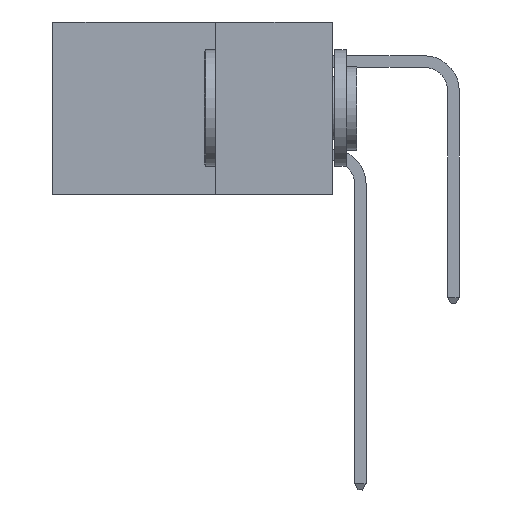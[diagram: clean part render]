
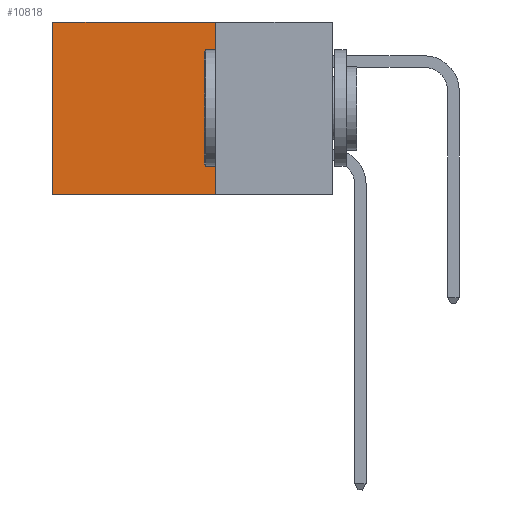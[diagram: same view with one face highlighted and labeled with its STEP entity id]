
A CAD part, left-side view. The second image highlights one B-rep face of the part: STEP entity #10818.
In plain terms, the highlighted planar face has unit normal (-1, 0, 0).
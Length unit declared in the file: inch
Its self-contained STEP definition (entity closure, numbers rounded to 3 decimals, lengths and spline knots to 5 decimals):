
#80 = VERTEX_POINT ( 'NONE', #12510 ) ;
#536 = FACE_OUTER_BOUND ( 'NONE', #19114, .T. ) ;
#728 = ORIENTED_EDGE ( 'NONE', *, *, #16095, .F. ) ;
#775 = VERTEX_POINT ( 'NONE', #17365 ) ;
#1237 = DIRECTION ( 'NONE',  ( 0., 0., -1. ) ) ;
#1368 = VECTOR ( 'NONE', #24370, 39.37008 ) ;
#1412 = LINE ( 'NONE', #24252, #15356 ) ;
#4120 = CARTESIAN_POINT ( 'NONE',  ( 0.298, 0.25, 0. ) ) ;
#4125 = DIRECTION ( 'NONE',  ( 0., 1., 0. ) ) ;
#4529 = CARTESIAN_POINT ( 'NONE',  ( 0.298, 0.6, -0.37 ) ) ;
#4601 = CARTESIAN_POINT ( 'NONE',  ( 0.298, 0.25, 0. ) ) ;
#5272 = ORIENTED_EDGE ( 'NONE', *, *, #18648, .T. ) ;
#6696 = VERTEX_POINT ( 'NONE', #4529 ) ;
#7100 = DIRECTION ( 'NONE',  ( 0., 1., 0. ) ) ;
#7927 = EDGE_CURVE ( 'NONE', #80, #16721, #14634, .T. ) ;
#8273 = ORIENTED_EDGE ( 'NONE', *, *, #7927, .F. ) ;
#9227 = EDGE_CURVE ( 'NONE', #80, #775, #24398, .T. ) ;
#9606 = AXIS2_PLACEMENT_3D ( 'NONE', #4120, #18722, #22922 ) ;
#10818 = ADVANCED_FACE ( 'NONE', ( #536 ), #14824, .F. ) ;
#11298 = VECTOR ( 'NONE', #4125, 39.37008 ) ;
#12510 = CARTESIAN_POINT ( 'NONE',  ( 0.298, 0.25, 0. ) ) ;
#13897 = ORIENTED_EDGE ( 'NONE', *, *, #9227, .T. ) ;
#14634 = LINE ( 'NONE', #4601, #20619 ) ;
#14824 = PLANE ( 'NONE',  #9606 ) ;
#15356 = VECTOR ( 'NONE', #7100, 39.37008 ) ;
#16095 = EDGE_CURVE ( 'NONE', #16721, #6696, #1412, .T. ) ;
#16721 = VERTEX_POINT ( 'NONE', #21459 ) ;
#17365 = CARTESIAN_POINT ( 'NONE',  ( 0.298, 0.6, 0. ) ) ;
#17786 = LINE ( 'NONE', #18844, #1368 ) ;
#18648 = EDGE_CURVE ( 'NONE', #775, #6696, #17786, .T. ) ;
#18722 = DIRECTION ( 'NONE',  ( 1., 0., 0. ) ) ;
#18844 = CARTESIAN_POINT ( 'NONE',  ( 0.298, 0.6, 0. ) ) ;
#19114 = EDGE_LOOP ( 'NONE', ( #5272, #728, #8273, #13897 ) ) ;
#19714 = CARTESIAN_POINT ( 'NONE',  ( 0.298, 0.25, 0. ) ) ;
#20619 = VECTOR ( 'NONE', #1237, 39.37008 ) ;
#21459 = CARTESIAN_POINT ( 'NONE',  ( 0.298, 0.25, -0.37 ) ) ;
#22922 = DIRECTION ( 'NONE',  ( 0., 0., -1. ) ) ;
#24252 = CARTESIAN_POINT ( 'NONE',  ( 0.298, 0.25, -0.37 ) ) ;
#24370 = DIRECTION ( 'NONE',  ( 0., 0., -1. ) ) ;
#24398 = LINE ( 'NONE', #19714, #11298 ) ;
